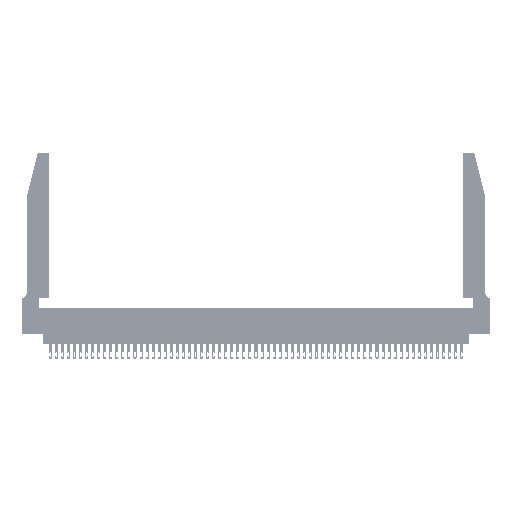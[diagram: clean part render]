
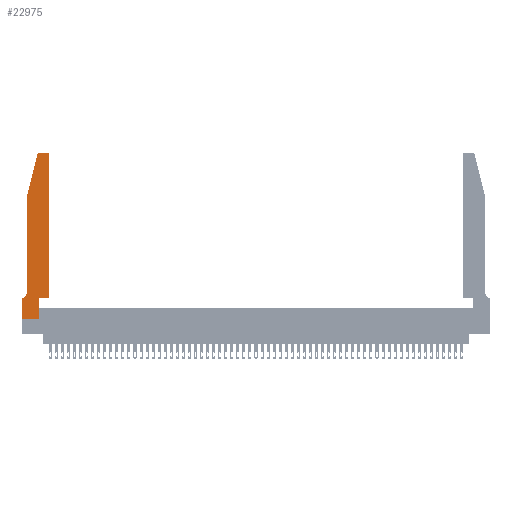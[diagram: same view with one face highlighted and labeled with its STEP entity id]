
A CAD part, top view. The second image highlights one B-rep face of the part: STEP entity #22975.
In plain terms, the highlighted planar face has unit normal (0, 0, 1).
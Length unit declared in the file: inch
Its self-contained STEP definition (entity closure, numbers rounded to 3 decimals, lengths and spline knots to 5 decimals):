
#338 = DIRECTION ( 'NONE',  ( 0., 0., 1. ) ) ;
#1086 = DIRECTION ( 'NONE',  ( -1., 0., 0. ) ) ;
#2561 = DIRECTION ( 'NONE',  ( 1., 0., 0. ) ) ;
#3504 = ORIENTED_EDGE ( 'NONE', *, *, #54683, .T. ) ;
#4664 = ORIENTED_EDGE ( 'NONE', *, *, #33616, .T. ) ;
#4809 = CARTESIAN_POINT ( 'NONE',  ( 0., 0.35, 0.37 ) ) ;
#5208 = VERTEX_POINT ( 'NONE', #10795 ) ;
#5384 = DIRECTION ( 'NONE',  ( -1., 0., 0. ) ) ;
#5481 = CARTESIAN_POINT ( 'NONE',  ( 0., 0., 0.37 ) ) ;
#5819 = DIRECTION ( 'NONE',  ( 0., 1., 0. ) ) ;
#6129 = DIRECTION ( 'NONE',  ( 0., 0., 1. ) ) ;
#6967 = CARTESIAN_POINT ( 'NONE',  ( 0.4505, 0.35, 0.37 ) ) ;
#7032 = LINE ( 'NONE', #53004, #23756 ) ;
#8006 = ORIENTED_EDGE ( 'NONE', *, *, #19364, .T. ) ;
#8060 = AXIS2_PLACEMENT_3D ( 'NONE', #11093, #28789, #28427 ) ;
#9101 = CARTESIAN_POINT ( 'NONE',  ( 0.0755, 2., 0.37 ) ) ;
#9510 = LINE ( 'NONE', #20879, #29493 ) ;
#10493 = VECTOR ( 'NONE', #49678, 39.37008 ) ;
#10631 = EDGE_CURVE ( 'NONE', #15841, #32856, #13181, .T. ) ;
#10795 = CARTESIAN_POINT ( 'NONE',  ( 0.25487, 2.72718, 0.37 ) ) ;
#10883 = VERTEX_POINT ( 'NONE', #47205 ) ;
#11093 = CARTESIAN_POINT ( 'NONE',  ( 0.4205, 2.72, 0.37 ) ) ;
#11373 = CIRCLE ( 'NONE', #11837, 0.07 ) ;
#11445 = VERTEX_POINT ( 'NONE', #29925 ) ;
#11500 = DIRECTION ( 'NONE',  ( -0.239, -0.971, 0. ) ) ;
#11512 = CARTESIAN_POINT ( 'NONE',  ( 0., 0., 0.37 ) ) ;
#11654 = VERTEX_POINT ( 'NONE', #27820 ) ;
#11832 = DIRECTION ( 'NONE',  ( 0., 1., 0. ) ) ;
#11837 = AXIS2_PLACEMENT_3D ( 'NONE', #52669, #14395, #1086 ) ;
#12031 = ORIENTED_EDGE ( 'NONE', *, *, #33704, .T. ) ;
#12402 = VECTOR ( 'NONE', #19580, 39.37008 ) ;
#13181 = LINE ( 'NONE', #45558, #10493 ) ;
#14395 = DIRECTION ( 'NONE',  ( 0., 0., -1. ) ) ;
#14793 = VERTEX_POINT ( 'NONE', #38746 ) ;
#14977 = AXIS2_PLACEMENT_3D ( 'NONE', #4809, #338, #43108 ) ;
#15695 = EDGE_LOOP ( 'NONE', ( #3504, #25390, #16734, #36810, #4664, #12031, #35484, #48510, #36690, #24595, #31428, #8006 ) ) ;
#15802 = CARTESIAN_POINT ( 'NONE',  ( 0.4205, 2.75, 0.37 ) ) ;
#15841 = VERTEX_POINT ( 'NONE', #25900 ) ;
#16734 = ORIENTED_EDGE ( 'NONE', *, *, #39359, .T. ) ;
#16772 = CARTESIAN_POINT ( 'NONE',  ( 0.4505, 2.72, 0.37 ) ) ;
#17371 = PLANE ( 'NONE',  #14977 ) ;
#17534 = CARTESIAN_POINT ( 'NONE',  ( 0.0055, 0.35, 0.37 ) ) ;
#17665 = VERTEX_POINT ( 'NONE', #17534 ) ;
#19159 = CARTESIAN_POINT ( 'NONE',  ( 0.0755, 2., 0.37 ) ) ;
#19364 = EDGE_CURVE ( 'NONE', #49803, #19462, #41870, .T. ) ;
#19462 = VERTEX_POINT ( 'NONE', #15802 ) ;
#19580 = DIRECTION ( 'NONE',  ( 1., 0., 0. ) ) ;
#20213 = LINE ( 'NONE', #6967, #38849 ) ;
#20879 = CARTESIAN_POINT ( 'NONE',  ( 0.2605, 2.75, 0.37 ) ) ;
#22221 = CARTESIAN_POINT ( 'NONE',  ( 0.0755, 0.35, 0.37 ) ) ;
#22975 = ADVANCED_FACE ( 'NONE', ( #48093 ), #17371, .T. ) ;
#23756 = VECTOR ( 'NONE', #11500, 39.37008 ) ;
#24595 = ORIENTED_EDGE ( 'NONE', *, *, #53718, .T. ) ;
#25390 = ORIENTED_EDGE ( 'NONE', *, *, #33860, .T. ) ;
#25900 = CARTESIAN_POINT ( 'NONE',  ( 0., 0.35, 0.37 ) ) ;
#26868 = VECTOR ( 'NONE', #11832, 39.37008 ) ;
#27820 = CARTESIAN_POINT ( 'NONE',  ( 0.4505, 0.35, 0.37 ) ) ;
#28262 = VECTOR ( 'NONE', #5819, 39.37008 ) ;
#28427 = DIRECTION ( 'NONE',  ( 1., 0., 0. ) ) ;
#28789 = DIRECTION ( 'NONE',  ( 0., 0., 1. ) ) ;
#28962 = DIRECTION ( 'NONE',  ( 1., 0., 0. ) ) ;
#29493 = VECTOR ( 'NONE', #47581, 39.37008 ) ;
#29770 = DIRECTION ( 'NONE',  ( 0., -1., 0. ) ) ;
#29925 = CARTESIAN_POINT ( 'NONE',  ( 0.0755, 0.42, 0.37 ) ) ;
#30492 = EDGE_CURVE ( 'NONE', #32856, #10883, #35758, .T. ) ;
#30937 = VERTEX_POINT ( 'NONE', #52750 ) ;
#31018 = VERTEX_POINT ( 'NONE', #19159 ) ;
#31349 = CARTESIAN_POINT ( 'NONE',  ( 0.2865, 0.35, 0.37 ) ) ;
#31428 = ORIENTED_EDGE ( 'NONE', *, *, #53652, .T. ) ;
#32856 = VERTEX_POINT ( 'NONE', #5481 ) ;
#33616 = EDGE_CURVE ( 'NONE', #11445, #17665, #11373, .T. ) ;
#33704 = EDGE_CURVE ( 'NONE', #17665, #15841, #43400, .T. ) ;
#33860 = EDGE_CURVE ( 'NONE', #14793, #5208, #48757, .T. ) ;
#35484 = ORIENTED_EDGE ( 'NONE', *, *, #10631, .T. ) ;
#35758 = LINE ( 'NONE', #11512, #12402 ) ;
#36690 = ORIENTED_EDGE ( 'NONE', *, *, #51814, .T. ) ;
#36810 = ORIENTED_EDGE ( 'NONE', *, *, #39064, .T. ) ;
#37108 = VECTOR ( 'NONE', #29770, 39.37008 ) ;
#38746 = CARTESIAN_POINT ( 'NONE',  ( 0.284, 2.75, 0.37 ) ) ;
#38849 = VECTOR ( 'NONE', #28962, 39.37008 ) ;
#39064 = EDGE_CURVE ( 'NONE', #31018, #11445, #45833, .T. ) ;
#39359 = EDGE_CURVE ( 'NONE', #5208, #31018, #7032, .T. ) ;
#40313 = LINE ( 'NONE', #31349, #28262 ) ;
#41870 = CIRCLE ( 'NONE', #8060, 0.03 ) ;
#43108 = DIRECTION ( 'NONE',  ( 1., 0., 0. ) ) ;
#43400 = LINE ( 'NONE', #22221, #45427 ) ;
#45427 = VECTOR ( 'NONE', #5384, 39.37008 ) ;
#45558 = CARTESIAN_POINT ( 'NONE',  ( 0., 0., 0.37 ) ) ;
#45833 = LINE ( 'NONE', #9101, #37108 ) ;
#47205 = CARTESIAN_POINT ( 'NONE',  ( 0.2865, 0., 0.37 ) ) ;
#47581 = DIRECTION ( 'NONE',  ( -1., 0., 0. ) ) ;
#48093 = FACE_OUTER_BOUND ( 'NONE', #15695, .T. ) ;
#48510 = ORIENTED_EDGE ( 'NONE', *, *, #30492, .T. ) ;
#48757 = CIRCLE ( 'NONE', #55118, 0.03 ) ;
#49450 = CARTESIAN_POINT ( 'NONE',  ( 0.284, 2.72, 0.37 ) ) ;
#49605 = LINE ( 'NONE', #54608, #26868 ) ;
#49678 = DIRECTION ( 'NONE',  ( 0., -1., 0. ) ) ;
#49803 = VERTEX_POINT ( 'NONE', #16772 ) ;
#51814 = EDGE_CURVE ( 'NONE', #10883, #30937, #40313, .T. ) ;
#52669 = CARTESIAN_POINT ( 'NONE',  ( 0.0055, 0.42, 0.37 ) ) ;
#52750 = CARTESIAN_POINT ( 'NONE',  ( 0.2865, 0.35, 0.37 ) ) ;
#53004 = CARTESIAN_POINT ( 'NONE',  ( 0.0755, 2., 0.37 ) ) ;
#53652 = EDGE_CURVE ( 'NONE', #11654, #49803, #49605, .T. ) ;
#53718 = EDGE_CURVE ( 'NONE', #30937, #11654, #20213, .T. ) ;
#54608 = CARTESIAN_POINT ( 'NONE',  ( 0.4505, 0.35, 0.37 ) ) ;
#54683 = EDGE_CURVE ( 'NONE', #19462, #14793, #9510, .T. ) ;
#55118 = AXIS2_PLACEMENT_3D ( 'NONE', #49450, #6129, #2561 ) ;
